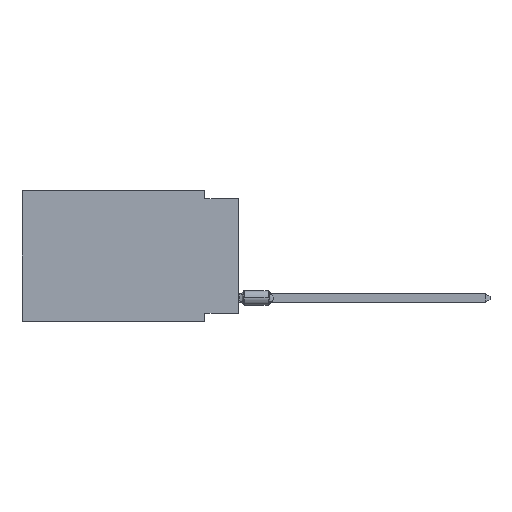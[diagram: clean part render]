
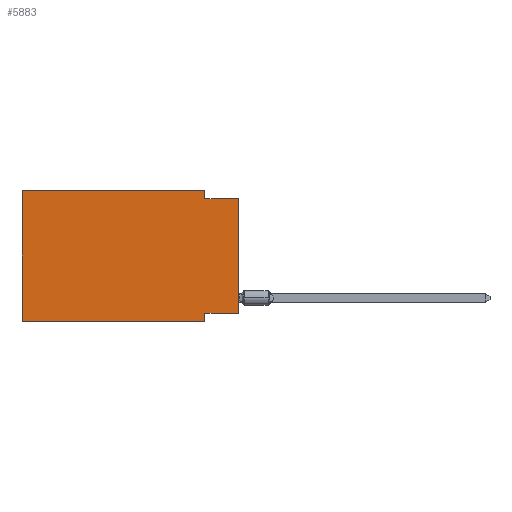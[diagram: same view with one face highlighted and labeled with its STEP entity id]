
A CAD part, left-side view. The second image highlights one B-rep face of the part: STEP entity #5883.
In plain terms, the highlighted planar face has unit normal (-1, 0, 0).
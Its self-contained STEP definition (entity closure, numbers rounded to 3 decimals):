
#158 = CARTESIAN_POINT ( 'NONE',  ( 0., 16.383, -9.906 ) ) ;
#437 = ORIENTED_EDGE ( 'NONE', *, *, #10064, .F. ) ;
#472 = LINE ( 'NONE', #4318, #5117 ) ;
#1403 = FACE_OUTER_BOUND ( 'NONE', #15594, .T. ) ;
#1517 = VECTOR ( 'NONE', #6243, 1000. ) ;
#1553 = ORIENTED_EDGE ( 'NONE', *, *, #5757, .T. ) ;
#1724 = ORIENTED_EDGE ( 'NONE', *, *, #2726, .F. ) ;
#1842 = VERTEX_POINT ( 'NONE', #12365 ) ;
#2377 = ORIENTED_EDGE ( 'NONE', *, *, #9176, .T. ) ;
#2726 = EDGE_CURVE ( 'NONE', #3564, #1842, #12154, .T. ) ;
#2739 = CARTESIAN_POINT ( 'NONE',  ( 0., 16.383, 0. ) ) ;
#2941 = DIRECTION ( 'NONE',  ( 0., 0., -1. ) ) ;
#3097 = ORIENTED_EDGE ( 'NONE', *, *, #3762, .F. ) ;
#3217 = LINE ( 'NONE', #13444, #5231 ) ;
#3377 = VERTEX_POINT ( 'NONE', #2739 ) ;
#3427 = VERTEX_POINT ( 'NONE', #158 ) ;
#3564 = VERTEX_POINT ( 'NONE', #5900 ) ;
#3762 = EDGE_CURVE ( 'NONE', #8173, #15215, #14318, .T. ) ;
#4035 = LINE ( 'NONE', #11980, #8722 ) ;
#4211 = DIRECTION ( 'NONE',  ( 0., -1., 0. ) ) ;
#4318 = CARTESIAN_POINT ( 'NONE',  ( 0., 16.383, -9.906 ) ) ;
#5117 = VECTOR ( 'NONE', #12074, 1000. ) ;
#5167 = CARTESIAN_POINT ( 'NONE',  ( 0., 0., -9.271 ) ) ;
#5180 = CARTESIAN_POINT ( 'NONE',  ( 0., 16.383, 0. ) ) ;
#5231 = VECTOR ( 'NONE', #9624, 1000. ) ;
#5235 = EDGE_CURVE ( 'NONE', #3377, #8347, #11793, .T. ) ;
#5284 = LINE ( 'NONE', #12957, #10820 ) ;
#5681 = VECTOR ( 'NONE', #4211, 1000. ) ;
#5757 = EDGE_CURVE ( 'NONE', #8173, #1842, #16634, .T. ) ;
#5784 = ORIENTED_EDGE ( 'NONE', *, *, #5235, .F. ) ;
#5883 = ADVANCED_FACE ( 'NONE', ( #1403 ), #9096, .F. ) ;
#5900 = CARTESIAN_POINT ( 'NONE',  ( 0., 2.54, -0.635 ) ) ;
#5944 = AXIS2_PLACEMENT_3D ( 'NONE', #5180, #6302, #11810 ) ;
#6122 = DIRECTION ( 'NONE',  ( 0., 0., 1. ) ) ;
#6243 = DIRECTION ( 'NONE',  ( 0., 1., 0. ) ) ;
#6302 = DIRECTION ( 'NONE',  ( 1., 0., 0. ) ) ;
#7222 = EDGE_CURVE ( 'NONE', #15215, #9574, #4035, .T. ) ;
#7627 = VECTOR ( 'NONE', #6122, 1000. ) ;
#8173 = VERTEX_POINT ( 'NONE', #5167 ) ;
#8347 = VERTEX_POINT ( 'NONE', #9513 ) ;
#8600 = CARTESIAN_POINT ( 'NONE',  ( 0., 0., 0. ) ) ;
#8722 = VECTOR ( 'NONE', #2941, 1000. ) ;
#9096 = PLANE ( 'NONE',  #5944 ) ;
#9176 = EDGE_CURVE ( 'NONE', #3427, #9574, #472, .T. ) ;
#9513 = CARTESIAN_POINT ( 'NONE',  ( 0., 2.54, 0. ) ) ;
#9574 = VERTEX_POINT ( 'NONE', #15258 ) ;
#9624 = DIRECTION ( 'NONE',  ( 0., 0., 1. ) ) ;
#10064 = EDGE_CURVE ( 'NONE', #3427, #3377, #3217, .T. ) ;
#10147 = CARTESIAN_POINT ( 'NONE',  ( 0., 0., -9.271 ) ) ;
#10765 = DIRECTION ( 'NONE',  ( 0., -1., 0. ) ) ;
#10820 = VECTOR ( 'NONE', #14419, 1000. ) ;
#11721 = CARTESIAN_POINT ( 'NONE',  ( 0., 16.383, 0. ) ) ;
#11793 = LINE ( 'NONE', #11721, #16846 ) ;
#11810 = DIRECTION ( 'NONE',  ( 0., 0., -1. ) ) ;
#11980 = CARTESIAN_POINT ( 'NONE',  ( 0., 2.54, -9.906 ) ) ;
#12074 = DIRECTION ( 'NONE',  ( 0., -1., 0. ) ) ;
#12154 = LINE ( 'NONE', #15906, #5681 ) ;
#12319 = EDGE_CURVE ( 'NONE', #8347, #3564, #5284, .T. ) ;
#12365 = CARTESIAN_POINT ( 'NONE',  ( 0., 0., -0.635 ) ) ;
#12428 = ORIENTED_EDGE ( 'NONE', *, *, #7222, .F. ) ;
#12957 = CARTESIAN_POINT ( 'NONE',  ( 0., 2.54, 0. ) ) ;
#13444 = CARTESIAN_POINT ( 'NONE',  ( 0., 16.383, 0. ) ) ;
#14318 = LINE ( 'NONE', #10147, #1517 ) ;
#14419 = DIRECTION ( 'NONE',  ( 0., 0., -1. ) ) ;
#14759 = ORIENTED_EDGE ( 'NONE', *, *, #12319, .F. ) ;
#15215 = VERTEX_POINT ( 'NONE', #16340 ) ;
#15258 = CARTESIAN_POINT ( 'NONE',  ( 0., 2.54, -9.906 ) ) ;
#15594 = EDGE_LOOP ( 'NONE', ( #1553, #1724, #14759, #5784, #437, #2377, #12428, #3097 ) ) ;
#15906 = CARTESIAN_POINT ( 'NONE',  ( 0., 0., -0.635 ) ) ;
#16340 = CARTESIAN_POINT ( 'NONE',  ( 0., 2.54, -9.271 ) ) ;
#16634 = LINE ( 'NONE', #8600, #7627 ) ;
#16846 = VECTOR ( 'NONE', #10765, 1000. ) ;
